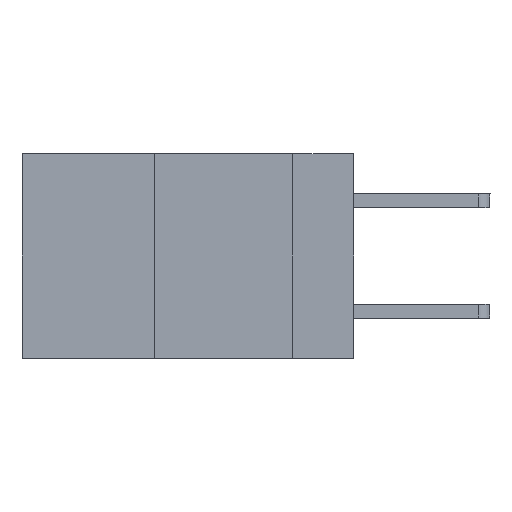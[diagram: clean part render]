
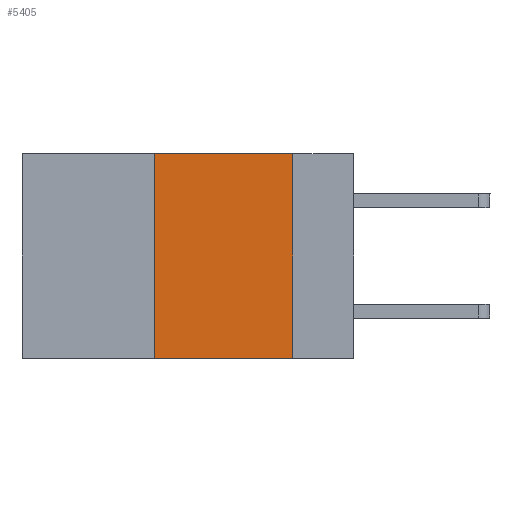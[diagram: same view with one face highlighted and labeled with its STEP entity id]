
A CAD part, left-side view. The second image highlights one B-rep face of the part: STEP entity #5405.
In plain terms, the highlighted planar face has unit normal (-1, 0, 0).
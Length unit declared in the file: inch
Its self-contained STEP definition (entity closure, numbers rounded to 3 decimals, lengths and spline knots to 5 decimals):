
#156 = DIRECTION ( 'NONE',  ( 0., 0., -1. ) ) ;
#208 = ORIENTED_EDGE ( 'NONE', *, *, #7216, .F. ) ;
#293 = VERTEX_POINT ( 'NONE', #1304 ) ;
#363 = CARTESIAN_POINT ( 'NONE',  ( 0., 0.36, 0. ) ) ;
#688 = VECTOR ( 'NONE', #9111, 39.37008 ) ;
#1304 = CARTESIAN_POINT ( 'NONE',  ( 0., 0.36, -0.37 ) ) ;
#1442 = ORIENTED_EDGE ( 'NONE', *, *, #9560, .T. ) ;
#1648 = VECTOR ( 'NONE', #5330, 39.37008 ) ;
#1667 = CARTESIAN_POINT ( 'NONE',  ( 0., 0.36, 0. ) ) ;
#1847 = CARTESIAN_POINT ( 'NONE',  ( 0., 0.6, -0.37 ) ) ;
#2240 = LINE ( 'NONE', #9038, #1648 ) ;
#2276 = DIRECTION ( 'NONE',  ( 0., 0., 1. ) ) ;
#2463 = VERTEX_POINT ( 'NONE', #3228 ) ;
#2758 = LINE ( 'NONE', #9774, #688 ) ;
#3228 = CARTESIAN_POINT ( 'NONE',  ( 0., 0.11, -0.37 ) ) ;
#3379 = DIRECTION ( 'NONE',  ( 1., 0., 0. ) ) ;
#3406 = EDGE_LOOP ( 'NONE', ( #208, #7854, #4142, #1442 ) ) ;
#3675 = EDGE_CURVE ( 'NONE', #293, #6811, #9997, .T. ) ;
#4142 = ORIENTED_EDGE ( 'NONE', *, *, #3675, .F. ) ;
#4624 = CARTESIAN_POINT ( 'NONE',  ( 0., 0.11, 0. ) ) ;
#4878 = DIRECTION ( 'NONE',  ( 0., -1., 0. ) ) ;
#5330 = DIRECTION ( 'NONE',  ( 0., 0., -1. ) ) ;
#5405 = ADVANCED_FACE ( 'NONE', ( #6319 ), #8852, .F. ) ;
#5761 = VECTOR ( 'NONE', #2276, 39.37008 ) ;
#6319 = FACE_OUTER_BOUND ( 'NONE', #3406, .T. ) ;
#6811 = VERTEX_POINT ( 'NONE', #363 ) ;
#7216 = EDGE_CURVE ( 'NONE', #9758, #2463, #2240, .T. ) ;
#7854 = ORIENTED_EDGE ( 'NONE', *, *, #8021, .F. ) ;
#7985 = LINE ( 'NONE', #1847, #9279 ) ;
#8021 = EDGE_CURVE ( 'NONE', #6811, #9758, #2758, .T. ) ;
#8807 = CARTESIAN_POINT ( 'NONE',  ( 0., 0.6, 0. ) ) ;
#8852 = PLANE ( 'NONE',  #8870 ) ;
#8870 = AXIS2_PLACEMENT_3D ( 'NONE', #8807, #3379, #156 ) ;
#9038 = CARTESIAN_POINT ( 'NONE',  ( 0., 0.11, 0. ) ) ;
#9111 = DIRECTION ( 'NONE',  ( 0., -1., 0. ) ) ;
#9279 = VECTOR ( 'NONE', #4878, 39.37008 ) ;
#9560 = EDGE_CURVE ( 'NONE', #293, #2463, #7985, .T. ) ;
#9758 = VERTEX_POINT ( 'NONE', #4624 ) ;
#9774 = CARTESIAN_POINT ( 'NONE',  ( 0., 0.6, 0. ) ) ;
#9997 = LINE ( 'NONE', #1667, #5761 ) ;
